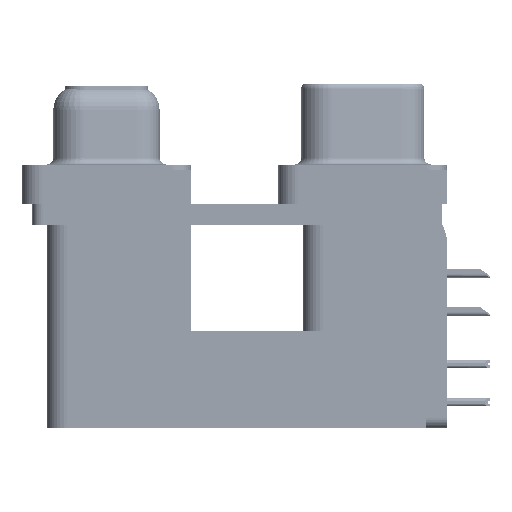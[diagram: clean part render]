
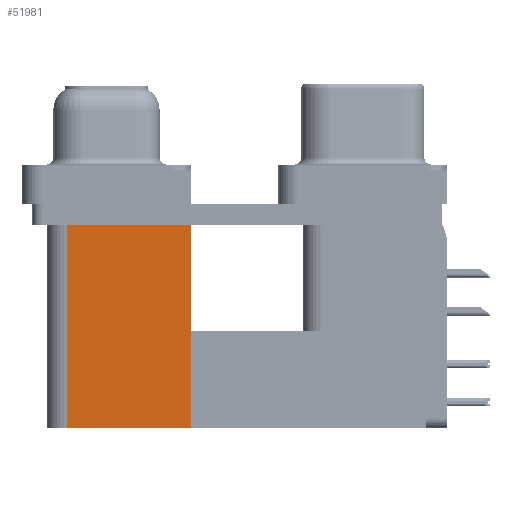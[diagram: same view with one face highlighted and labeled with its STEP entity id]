
A CAD part, left-side view. The second image highlights one B-rep face of the part: STEP entity #51981.
In plain terms, the highlighted planar face has unit normal (-1, 0, 0).
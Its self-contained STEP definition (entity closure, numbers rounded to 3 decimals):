
#707 = VERTEX_POINT ( 'NONE', #39522 ) ;
#1208 = LINE ( 'NONE', #58033, #15387 ) ;
#3700 = DIRECTION ( 'NONE',  ( 0., 1., 0. ) ) ;
#4733 = ORIENTED_EDGE ( 'NONE', *, *, #56562, .T. ) ;
#5234 = ORIENTED_EDGE ( 'NONE', *, *, #45819, .F. ) ;
#9625 = CARTESIAN_POINT ( 'NONE',  ( 3.79, 12.775, -19.2 ) ) ;
#11678 = AXIS2_PLACEMENT_3D ( 'NONE', #25246, #46148, #3700 ) ;
#14086 = LINE ( 'NONE', #61298, #15511 ) ;
#15387 = VECTOR ( 'NONE', #32387, 1000. ) ;
#15511 = VECTOR ( 'NONE', #66114, 1000. ) ;
#19745 = CARTESIAN_POINT ( 'NONE',  ( 3.79, 12.775, -2.5 ) ) ;
#22260 = ORIENTED_EDGE ( 'NONE', *, *, #65164, .T. ) ;
#25246 = CARTESIAN_POINT ( 'NONE',  ( 3.79, 12.775, -19.2 ) ) ;
#25381 = LINE ( 'NONE', #9625, #61421 ) ;
#32387 = DIRECTION ( 'NONE',  ( 0., 1., 0. ) ) ;
#36596 = VERTEX_POINT ( 'NONE', #64314 ) ;
#39120 = VERTEX_POINT ( 'NONE', #19745 ) ;
#39522 = CARTESIAN_POINT ( 'NONE',  ( 3.79, 21.975, -2.5 ) ) ;
#40348 = FACE_OUTER_BOUND ( 'NONE', #63818, .T. ) ;
#45819 = EDGE_CURVE ( 'NONE', #36596, #707, #54137, .T. ) ;
#46148 = DIRECTION ( 'NONE',  ( 1., 0., 0. ) ) ;
#50995 = VECTOR ( 'NONE', #64389, 1000. ) ;
#51981 = ADVANCED_FACE ( 'NONE', ( #40348 ), #56053, .F. ) ;
#52073 = DIRECTION ( 'NONE',  ( 0., 0., 1. ) ) ;
#54137 = LINE ( 'NONE', #59596, #50995 ) ;
#54477 = VERTEX_POINT ( 'NONE', #63333 ) ;
#56053 = PLANE ( 'NONE',  #11678 ) ;
#56562 = EDGE_CURVE ( 'NONE', #39120, #707, #1208, .T. ) ;
#58033 = CARTESIAN_POINT ( 'NONE',  ( 3.79, 12.775, -2.5 ) ) ;
#59596 = CARTESIAN_POINT ( 'NONE',  ( 3.79, 21.975, -19.2 ) ) ;
#59621 = ORIENTED_EDGE ( 'NONE', *, *, #64920, .F. ) ;
#61298 = CARTESIAN_POINT ( 'NONE',  ( 3.79, 12.775, -19.2 ) ) ;
#61421 = VECTOR ( 'NONE', #52073, 1000. ) ;
#63333 = CARTESIAN_POINT ( 'NONE',  ( 3.79, 12.775, -19.2 ) ) ;
#63818 = EDGE_LOOP ( 'NONE', ( #4733, #5234, #59621, #22260 ) ) ;
#64314 = CARTESIAN_POINT ( 'NONE',  ( 3.79, 21.975, -19.2 ) ) ;
#64389 = DIRECTION ( 'NONE',  ( 0., 0., 1. ) ) ;
#64920 = EDGE_CURVE ( 'NONE', #54477, #36596, #14086, .T. ) ;
#65164 = EDGE_CURVE ( 'NONE', #54477, #39120, #25381, .T. ) ;
#66114 = DIRECTION ( 'NONE',  ( 0., 1., 0. ) ) ;
